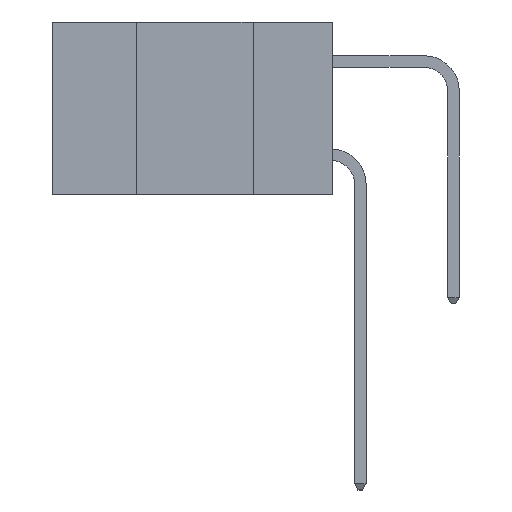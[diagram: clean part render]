
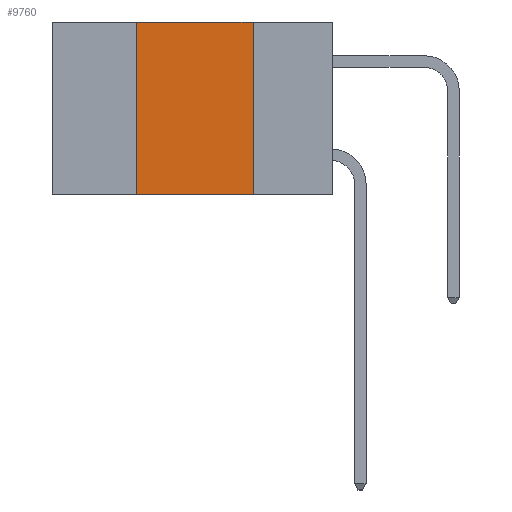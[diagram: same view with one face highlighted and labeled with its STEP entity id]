
A CAD part, left-side view. The second image highlights one B-rep face of the part: STEP entity #9760.
In plain terms, the highlighted planar face has unit normal (-1, 0, 0).
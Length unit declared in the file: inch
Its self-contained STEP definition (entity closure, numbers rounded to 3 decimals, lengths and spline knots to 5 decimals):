
#139 = VERTEX_POINT ( 'NONE', #3147 ) ;
#550 = ORIENTED_EDGE ( 'NONE', *, *, #4074, .F. ) ;
#773 = EDGE_CURVE ( 'NONE', #139, #5174, #4079, .T. ) ;
#3147 = CARTESIAN_POINT ( 'NONE',  ( 0., 0.17, 0. ) ) ;
#3303 = AXIS2_PLACEMENT_3D ( 'NONE', #9880, #8947, #9276 ) ;
#3649 = CARTESIAN_POINT ( 'NONE',  ( 0., 0.17, -0.37 ) ) ;
#4011 = ORIENTED_EDGE ( 'NONE', *, *, #773, .F. ) ;
#4074 = EDGE_CURVE ( 'NONE', #9775, #10416, #5915, .T. ) ;
#4079 = LINE ( 'NONE', #11396, #6963 ) ;
#4187 = FACE_OUTER_BOUND ( 'NONE', #14347, .T. ) ;
#5022 = VECTOR ( 'NONE', #12512, 39.37008 ) ;
#5131 = VECTOR ( 'NONE', #11420, 39.37008 ) ;
#5174 = VERTEX_POINT ( 'NONE', #3649 ) ;
#5902 = LINE ( 'NONE', #15000, #11947 ) ;
#5915 = LINE ( 'NONE', #11385, #5131 ) ;
#6317 = DIRECTION ( 'NONE',  ( 0., -1., 0. ) ) ;
#6349 = ORIENTED_EDGE ( 'NONE', *, *, #9801, .T. ) ;
#6963 = VECTOR ( 'NONE', #11414, 39.37008 ) ;
#7360 = EDGE_CURVE ( 'NONE', #10416, #139, #14224, .T. ) ;
#8048 = CARTESIAN_POINT ( 'NONE',  ( 0., 0.42, 0. ) ) ;
#8206 = CARTESIAN_POINT ( 'NONE',  ( 0., 0.42, -0.37 ) ) ;
#8947 = DIRECTION ( 'NONE',  ( 1., 0., 0. ) ) ;
#9276 = DIRECTION ( 'NONE',  ( 0., 0., -1. ) ) ;
#9640 = PLANE ( 'NONE',  #3303 ) ;
#9760 = ADVANCED_FACE ( 'NONE', ( #4187 ), #9640, .F. ) ;
#9775 = VERTEX_POINT ( 'NONE', #8206 ) ;
#9801 = EDGE_CURVE ( 'NONE', #9775, #5174, #5902, .T. ) ;
#9880 = CARTESIAN_POINT ( 'NONE',  ( 0., 0.6, 0. ) ) ;
#10416 = VERTEX_POINT ( 'NONE', #8048 ) ;
#11385 = CARTESIAN_POINT ( 'NONE',  ( 0., 0.42, -0.37 ) ) ;
#11396 = CARTESIAN_POINT ( 'NONE',  ( 0., 0.17, -0.37 ) ) ;
#11414 = DIRECTION ( 'NONE',  ( 0., 0., -1. ) ) ;
#11420 = DIRECTION ( 'NONE',  ( 0., 0., 1. ) ) ;
#11947 = VECTOR ( 'NONE', #6317, 39.37008 ) ;
#12512 = DIRECTION ( 'NONE',  ( 0., -1., 0. ) ) ;
#12541 = ORIENTED_EDGE ( 'NONE', *, *, #7360, .F. ) ;
#12595 = CARTESIAN_POINT ( 'NONE',  ( 0., 0.6, 0. ) ) ;
#14224 = LINE ( 'NONE', #12595, #5022 ) ;
#14347 = EDGE_LOOP ( 'NONE', ( #4011, #12541, #550, #6349 ) ) ;
#15000 = CARTESIAN_POINT ( 'NONE',  ( 0., 0.6, -0.37 ) ) ;
